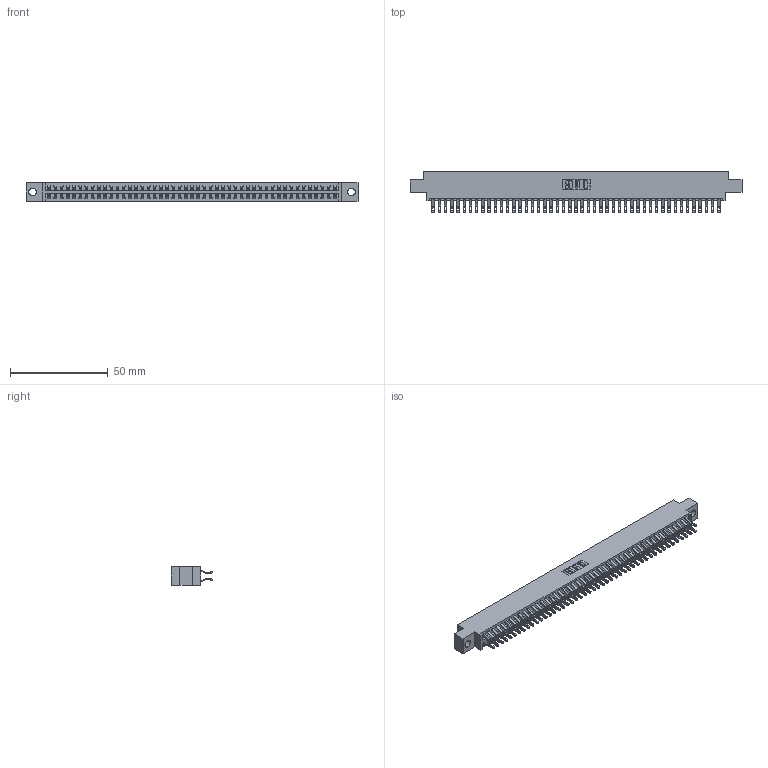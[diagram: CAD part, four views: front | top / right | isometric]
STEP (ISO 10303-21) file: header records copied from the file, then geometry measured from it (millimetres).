
FILE_DESCRIPTION (( 'STEP AP203' ), '1' );
FILE_NAME ('346-094-555-804.STEP', '2022-05-26T14:55:29', ( '' ), ( '' ), 'SwSTEP 2.0', 'SolidWorks 2020', '' );
FILE_SCHEMA (( 'CONFIG_CONTROL_DESIGN' ));
Length unit declared in the file: inch
Products named in the file (3): 346 Part_0.170 Offset - 0.156 Dia-TH; 345-292-001_555 Tail; 346-094-555-804
Assembly tree (95 placements, depth 2):
  346-094-555-804
    346 Part_0.170 Offset - 0.156 Dia-TH
    345-292-001_555 Tail  x94
Bounding box: 169.8 x 21.46 x 9.4 mm (x, y, z)
Volume: 16608.4 mm3; surface area: 23907.4 mm2
Topology: 95 solids, 95 shells, 5592 faces, 17579 edges, 11718 vertices
Faces by surface type: plane 3196, cylinder 2396
Entity records: 30877 total; most frequent: CARTESIAN_POINT 5124, ORIENTED_EDGE 5026, DIRECTION 4533, EDGE_CURVE 2513, VECTOR 2173, LINE 2173, VERTEX_POINT 1674, AXIS2_PLACEMENT_3D 1180
